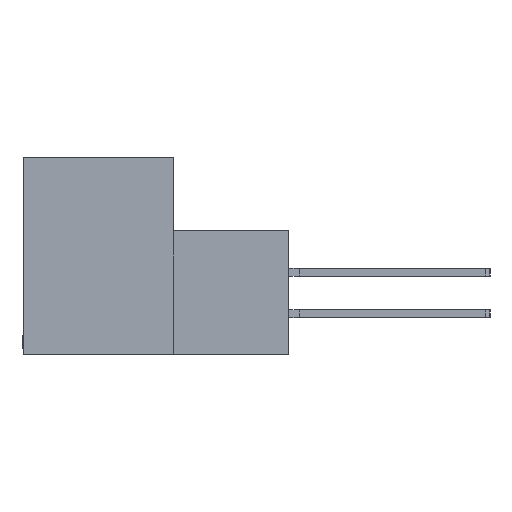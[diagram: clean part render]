
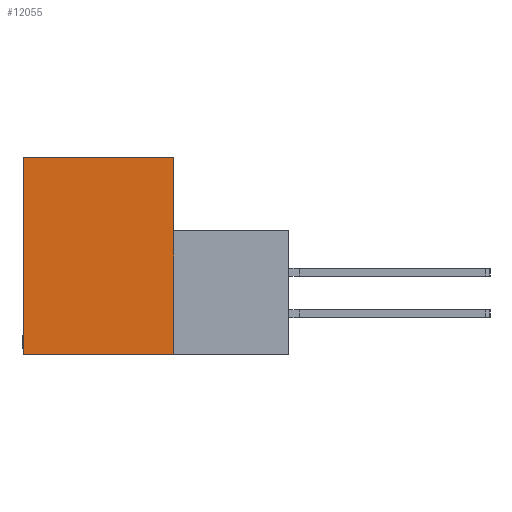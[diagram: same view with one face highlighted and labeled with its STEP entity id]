
A CAD part, left-side view. The second image highlights one B-rep face of the part: STEP entity #12055.
In plain terms, the highlighted planar face has unit normal (-1, 0, 0).
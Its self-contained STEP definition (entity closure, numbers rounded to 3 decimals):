
#1781 = EDGE_CURVE ( 'NONE', #42857, #40268, #50155, .T. ) ;
#6110 = ORIENTED_EDGE ( 'NONE', *, *, #1781, .F. ) ;
#8004 = CARTESIAN_POINT ( 'NONE',  ( 0., -8.814, -15.088 ) ) ;
#8374 = CARTESIAN_POINT ( 'NONE',  ( 0., 11.506, 0. ) ) ;
#8720 = VECTOR ( 'NONE', #48342, 1000. ) ;
#9338 = ORIENTED_EDGE ( 'NONE', *, *, #16573, .F. ) ;
#10840 = EDGE_CURVE ( 'NONE', #25445, #42857, #28367, .T. ) ;
#12055 = ADVANCED_FACE ( 'NONE', ( #40586 ), #20297, .F. ) ;
#16573 = EDGE_CURVE ( 'NONE', #40268, #43215, #46415, .T. ) ;
#19727 = DIRECTION ( 'NONE',  ( 0., -1., 0. ) ) ;
#19956 = DIRECTION ( 'NONE',  ( 1., 0., 0. ) ) ;
#20297 = PLANE ( 'NONE',  #42382 ) ;
#24355 = DIRECTION ( 'NONE',  ( 0., 0., -1. ) ) ;
#24535 = CARTESIAN_POINT ( 'NONE',  ( 0., 11.506, -15.088 ) ) ;
#25445 = VERTEX_POINT ( 'NONE', #26321 ) ;
#25861 = LINE ( 'NONE', #8374, #32568 ) ;
#26321 = CARTESIAN_POINT ( 'NONE',  ( 0., 0., 0. ) ) ;
#28367 = LINE ( 'NONE', #48497, #38217 ) ;
#29014 = CARTESIAN_POINT ( 'NONE',  ( 0., 11.506, -15.088 ) ) ;
#31580 = VECTOR ( 'NONE', #43219, 1000. ) ;
#31688 = DIRECTION ( 'NONE',  ( 0., 0., -1. ) ) ;
#32568 = VECTOR ( 'NONE', #19727, 1000. ) ;
#35753 = EDGE_LOOP ( 'NONE', ( #6110, #39694, #41851, #9338 ) ) ;
#38217 = VECTOR ( 'NONE', #24355, 1000. ) ;
#39694 = ORIENTED_EDGE ( 'NONE', *, *, #10840, .F. ) ;
#40073 = CARTESIAN_POINT ( 'NONE',  ( 0., 0., -15.088 ) ) ;
#40268 = VERTEX_POINT ( 'NONE', #29014 ) ;
#40321 = CARTESIAN_POINT ( 'NONE',  ( 0., 0., 0. ) ) ;
#40586 = FACE_OUTER_BOUND ( 'NONE', #35753, .T. ) ;
#41851 = ORIENTED_EDGE ( 'NONE', *, *, #44454, .F. ) ;
#42382 = AXIS2_PLACEMENT_3D ( 'NONE', #40321, #19956, #31688 ) ;
#42857 = VERTEX_POINT ( 'NONE', #40073 ) ;
#43215 = VERTEX_POINT ( 'NONE', #50787 ) ;
#43219 = DIRECTION ( 'NONE',  ( 0., 1., 0. ) ) ;
#44454 = EDGE_CURVE ( 'NONE', #43215, #25445, #25861, .T. ) ;
#46415 = LINE ( 'NONE', #24535, #8720 ) ;
#48342 = DIRECTION ( 'NONE',  ( 0., 0., 1. ) ) ;
#48497 = CARTESIAN_POINT ( 'NONE',  ( 0., 0., 0. ) ) ;
#50155 = LINE ( 'NONE', #8004, #31580 ) ;
#50787 = CARTESIAN_POINT ( 'NONE',  ( 0., 11.506, 0. ) ) ;
